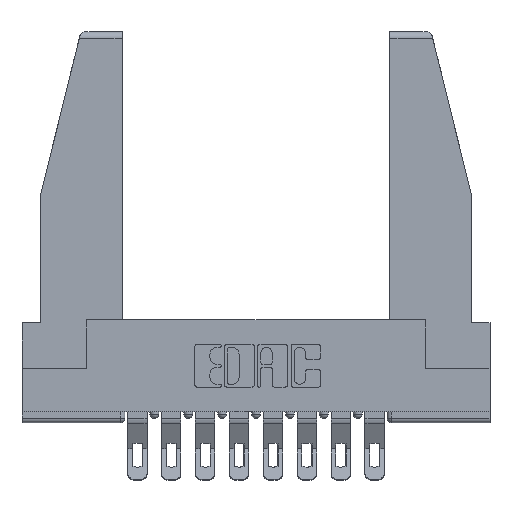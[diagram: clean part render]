
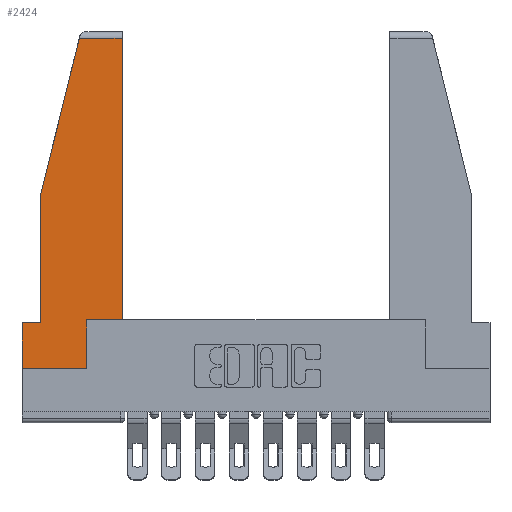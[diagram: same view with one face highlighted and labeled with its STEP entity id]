
A CAD part, top view. The second image highlights one B-rep face of the part: STEP entity #2424.
In plain terms, the highlighted planar face has unit normal (0, 0, 1).
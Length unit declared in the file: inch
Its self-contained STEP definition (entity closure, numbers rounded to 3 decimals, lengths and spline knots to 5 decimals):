
#2 = VECTOR ( 'NONE', #10146, 39.37008 ) ;
#181 = DIRECTION ( 'NONE',  ( -1., 0., 0. ) ) ;
#619 = CARTESIAN_POINT ( 'NONE',  ( 0.2636, 1.52, 0. ) ) ;
#875 = EDGE_CURVE ( 'NONE', #5630, #11874, #13828, .T. ) ;
#955 = LINE ( 'NONE', #2513, #12680 ) ;
#981 = ORIENTED_EDGE ( 'NONE', *, *, #7187, .T. ) ;
#1065 = LINE ( 'NONE', #2977, #13484 ) ;
#1162 = CARTESIAN_POINT ( 'NONE',  ( 0., 0., 0. ) ) ;
#1195 = PLANE ( 'NONE',  #6610 ) ;
#1566 = ORIENTED_EDGE ( 'NONE', *, *, #1804, .T. ) ;
#1790 = CARTESIAN_POINT ( 'NONE',  ( 0.086, 0.21, 0. ) ) ;
#1804 = EDGE_CURVE ( 'NONE', #11874, #11274, #2260, .T. ) ;
#1825 = CARTESIAN_POINT ( 'NONE',  ( 0.461, 0.223, 0. ) ) ;
#1849 = VERTEX_POINT ( 'NONE', #12441 ) ;
#2260 = LINE ( 'NONE', #1162, #13276 ) ;
#2424 = ADVANCED_FACE ( 'NONE', ( #7380 ), #1195, .T. ) ;
#2513 = CARTESIAN_POINT ( 'NONE',  ( 0., 0.21, 0. ) ) ;
#2558 = ORIENTED_EDGE ( 'NONE', *, *, #7020, .T. ) ;
#2802 = EDGE_CURVE ( 'NONE', #1849, #3428, #7873, .T. ) ;
#2820 = VERTEX_POINT ( 'NONE', #619 ) ;
#2977 = CARTESIAN_POINT ( 'NONE',  ( 0., 1.52, 0. ) ) ;
#3159 = DIRECTION ( 'NONE',  ( 0., 1., 0. ) ) ;
#3228 = DIRECTION ( 'NONE',  ( 0., -1., 0. ) ) ;
#3428 = VERTEX_POINT ( 'NONE', #14234 ) ;
#4258 = CARTESIAN_POINT ( 'NONE',  ( 0.086, 0.8, 0. ) ) ;
#4648 = VERTEX_POINT ( 'NONE', #4852 ) ;
#4839 = LINE ( 'NONE', #5310, #7056 ) ;
#4852 = CARTESIAN_POINT ( 'NONE',  ( 0.086, 0.8, 0. ) ) ;
#5186 = EDGE_CURVE ( 'NONE', #6070, #5630, #955, .T. ) ;
#5310 = CARTESIAN_POINT ( 'NONE',  ( 0.271, 1.55, 0. ) ) ;
#5630 = VERTEX_POINT ( 'NONE', #11602 ) ;
#6070 = VERTEX_POINT ( 'NONE', #1790 ) ;
#6205 = ORIENTED_EDGE ( 'NONE', *, *, #875, .T. ) ;
#6300 = ORIENTED_EDGE ( 'NONE', *, *, #13510, .T. ) ;
#6336 = CARTESIAN_POINT ( 'NONE',  ( 0.297, 0., 0. ) ) ;
#6406 = DIRECTION ( 'NONE',  ( -0.239, -0.971, 0. ) ) ;
#6610 = AXIS2_PLACEMENT_3D ( 'NONE', #13380, #12378, #10186 ) ;
#7020 = EDGE_CURVE ( 'NONE', #3428, #2820, #1065, .T. ) ;
#7056 = VECTOR ( 'NONE', #6406, 39.37008 ) ;
#7187 = EDGE_CURVE ( 'NONE', #2820, #4648, #4839, .T. ) ;
#7380 = FACE_OUTER_BOUND ( 'NONE', #7838, .T. ) ;
#7838 = EDGE_LOOP ( 'NONE', ( #12914, #2558, #981, #12133, #9951, #6205, #1566, #6300, #12671 ) ) ;
#7873 = LINE ( 'NONE', #1825, #12738 ) ;
#8846 = CARTESIAN_POINT ( 'NONE',  ( 0.297, 0.223, 0. ) ) ;
#8852 = DIRECTION ( 'NONE',  ( 1., 0., 0. ) ) ;
#9566 = DIRECTION ( 'NONE',  ( 1., 0., 0. ) ) ;
#9615 = CARTESIAN_POINT ( 'NONE',  ( 0.297, 0.223, 0. ) ) ;
#9670 = VECTOR ( 'NONE', #3228, 39.37008 ) ;
#9951 = ORIENTED_EDGE ( 'NONE', *, *, #5186, .T. ) ;
#10144 = VECTOR ( 'NONE', #13733, 39.37008 ) ;
#10146 = DIRECTION ( 'NONE',  ( 0., -1., 0. ) ) ;
#10186 = DIRECTION ( 'NONE',  ( 1., 0., 0. ) ) ;
#10798 = CARTESIAN_POINT ( 'NONE',  ( 0., 0., 0. ) ) ;
#11274 = VERTEX_POINT ( 'NONE', #6336 ) ;
#11602 = CARTESIAN_POINT ( 'NONE',  ( 0., 0.21, 0. ) ) ;
#11804 = DIRECTION ( 'NONE',  ( -1., 0., 0. ) ) ;
#11874 = VERTEX_POINT ( 'NONE', #10798 ) ;
#12133 = ORIENTED_EDGE ( 'NONE', *, *, #14310, .T. ) ;
#12292 = CARTESIAN_POINT ( 'NONE',  ( 0., 0.21, 0. ) ) ;
#12378 = DIRECTION ( 'NONE',  ( 0., 0., 1. ) ) ;
#12441 = CARTESIAN_POINT ( 'NONE',  ( 0.461, 0.223, 0. ) ) ;
#12671 = ORIENTED_EDGE ( 'NONE', *, *, #13027, .T. ) ;
#12676 = LINE ( 'NONE', #9615, #13887 ) ;
#12680 = VECTOR ( 'NONE', #181, 39.37008 ) ;
#12738 = VECTOR ( 'NONE', #3159, 39.37008 ) ;
#12914 = ORIENTED_EDGE ( 'NONE', *, *, #2802, .T. ) ;
#12945 = LINE ( 'NONE', #13648, #10144 ) ;
#13027 = EDGE_CURVE ( 'NONE', #13193, #1849, #12676, .T. ) ;
#13193 = VERTEX_POINT ( 'NONE', #8846 ) ;
#13276 = VECTOR ( 'NONE', #8852, 39.37008 ) ;
#13288 = LINE ( 'NONE', #4258, #9670 ) ;
#13380 = CARTESIAN_POINT ( 'NONE',  ( 0., 0., 0. ) ) ;
#13484 = VECTOR ( 'NONE', #11804, 39.37008 ) ;
#13510 = EDGE_CURVE ( 'NONE', #11274, #13193, #12945, .T. ) ;
#13648 = CARTESIAN_POINT ( 'NONE',  ( 0.297, 0., 0. ) ) ;
#13733 = DIRECTION ( 'NONE',  ( 0., 1., 0. ) ) ;
#13828 = LINE ( 'NONE', #12292, #2 ) ;
#13887 = VECTOR ( 'NONE', #9566, 39.37008 ) ;
#14234 = CARTESIAN_POINT ( 'NONE',  ( 0.461, 1.52, 0. ) ) ;
#14310 = EDGE_CURVE ( 'NONE', #4648, #6070, #13288, .T. ) ;
